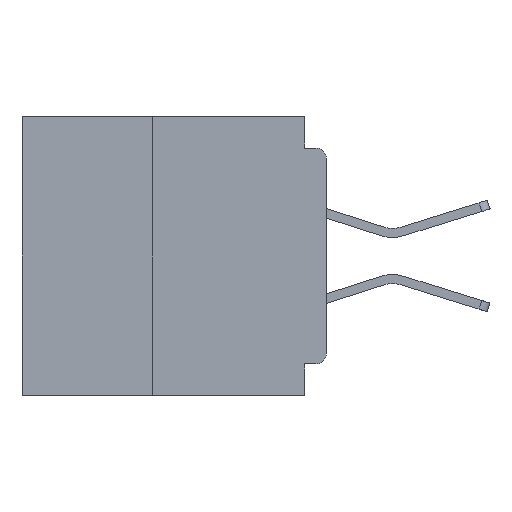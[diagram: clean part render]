
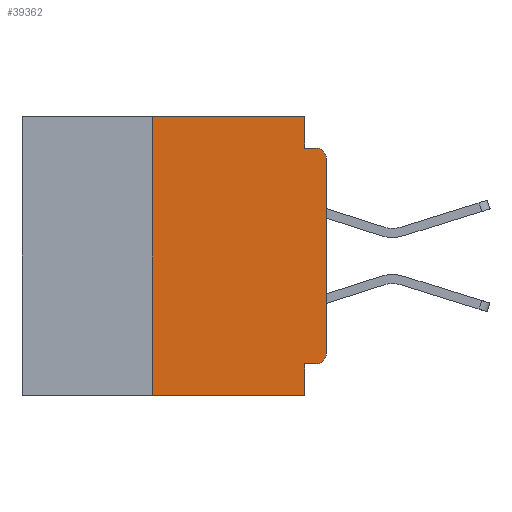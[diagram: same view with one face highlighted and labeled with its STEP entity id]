
A CAD part, left-side view. The second image highlights one B-rep face of the part: STEP entity #39362.
In plain terms, the highlighted planar face has unit normal (-1, 0, 0).
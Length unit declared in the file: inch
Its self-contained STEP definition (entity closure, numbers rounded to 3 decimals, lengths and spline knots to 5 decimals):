
#605 = DIRECTION ( 'NONE',  ( -1., 0., 0. ) ) ;
#1398 = CARTESIAN_POINT ( 'NONE',  ( 0., 0.25, 0. ) ) ;
#1966 = EDGE_CURVE ( 'NONE', #12375, #39930, #5953, .T. ) ;
#2686 = CARTESIAN_POINT ( 'NONE',  ( 0., 0., 0. ) ) ;
#2835 = ORIENTED_EDGE ( 'NONE', *, *, #18315, .T. ) ;
#3194 = DIRECTION ( 'NONE',  ( 0., 1., 0. ) ) ;
#5110 = CARTESIAN_POINT ( 'NONE',  ( 0., 0.25, -0.4 ) ) ;
#5703 = LINE ( 'NONE', #2686, #30418 ) ;
#5946 = AXIS2_PLACEMENT_3D ( 'NONE', #6601, #29172, #9844 ) ;
#5953 = LINE ( 'NONE', #39420, #28648 ) ;
#6601 = CARTESIAN_POINT ( 'NONE',  ( 0., 0.015, -0.34 ) ) ;
#7279 = ORIENTED_EDGE ( 'NONE', *, *, #30852, .F. ) ;
#7364 = PLANE ( 'NONE',  #23632 ) ;
#9844 = DIRECTION ( 'NONE',  ( 0., 0., -1. ) ) ;
#10402 = VECTOR ( 'NONE', #3194, 39.37008 ) ;
#10815 = EDGE_CURVE ( 'NONE', #17379, #29961, #40975, .T. ) ;
#10957 = ORIENTED_EDGE ( 'NONE', *, *, #1966, .T. ) ;
#11171 = ORIENTED_EDGE ( 'NONE', *, *, #10815, .T. ) ;
#11207 = EDGE_CURVE ( 'NONE', #12375, #24664, #19325, .T. ) ;
#12375 = VERTEX_POINT ( 'NONE', #5110 ) ;
#13879 = DIRECTION ( 'NONE',  ( 0., 0., -1. ) ) ;
#14001 = VECTOR ( 'NONE', #37225, 39.37008 ) ;
#14435 = ORIENTED_EDGE ( 'NONE', *, *, #35117, .F. ) ;
#15140 = CARTESIAN_POINT ( 'NONE',  ( 0., 0., -0.34 ) ) ;
#15181 = ORIENTED_EDGE ( 'NONE', *, *, #16352, .F. ) ;
#15329 = VERTEX_POINT ( 'NONE', #35336 ) ;
#15531 = CIRCLE ( 'NONE', #5946, 0.015 ) ;
#15926 = FACE_OUTER_BOUND ( 'NONE', #25054, .T. ) ;
#16352 = EDGE_CURVE ( 'NONE', #31308, #29961, #40665, .T. ) ;
#17379 = VERTEX_POINT ( 'NONE', #39952 ) ;
#18208 = VERTEX_POINT ( 'NONE', #15140 ) ;
#18305 = VECTOR ( 'NONE', #28153, 39.37008 ) ;
#18315 = EDGE_CURVE ( 'NONE', #18208, #17379, #5703, .T. ) ;
#18844 = VECTOR ( 'NONE', #39187, 39.37008 ) ;
#19325 = LINE ( 'NONE', #24911, #18305 ) ;
#19331 = CARTESIAN_POINT ( 'NONE',  ( 0., 0.031, -0.045 ) ) ;
#19873 = CARTESIAN_POINT ( 'NONE',  ( 0., 0.031, -0.4 ) ) ;
#19899 = CARTESIAN_POINT ( 'NONE',  ( 0., 0.015, -0.06 ) ) ;
#22555 = EDGE_CURVE ( 'NONE', #22811, #18208, #15531, .T. ) ;
#22563 = ORIENTED_EDGE ( 'NONE', *, *, #11207, .F. ) ;
#22811 = VERTEX_POINT ( 'NONE', #23915 ) ;
#23142 = DIRECTION ( 'NONE',  ( 0., 0., -1. ) ) ;
#23632 = AXIS2_PLACEMENT_3D ( 'NONE', #29913, #33124, #13879 ) ;
#23915 = CARTESIAN_POINT ( 'NONE',  ( 0., 0.015, -0.355 ) ) ;
#24546 = DIRECTION ( 'NONE',  ( 0., -1., 0. ) ) ;
#24607 = VECTOR ( 'NONE', #32997, 39.37008 ) ;
#24664 = VERTEX_POINT ( 'NONE', #1398 ) ;
#24735 = CARTESIAN_POINT ( 'NONE',  ( 0., 0.015, -0.045 ) ) ;
#24911 = CARTESIAN_POINT ( 'NONE',  ( 0., 0.25, -0.4 ) ) ;
#25054 = EDGE_LOOP ( 'NONE', ( #2835, #11171, #15181, #36501, #30398, #22563, #10957, #7279, #14435, #37507 ) ) ;
#25589 = LINE ( 'NONE', #29792, #24607 ) ;
#25751 = CARTESIAN_POINT ( 'NONE',  ( 0., 0.031, 0. ) ) ;
#27282 = VECTOR ( 'NONE', #24546, 39.37008 ) ;
#28153 = DIRECTION ( 'NONE',  ( 0., 0., 1. ) ) ;
#28418 = LINE ( 'NONE', #35930, #18844 ) ;
#28648 = VECTOR ( 'NONE', #38676, 39.37008 ) ;
#28766 = EDGE_CURVE ( 'NONE', #24664, #39794, #35855, .T. ) ;
#29172 = DIRECTION ( 'NONE',  ( -1., 0., 0. ) ) ;
#29792 = CARTESIAN_POINT ( 'NONE',  ( 0., 0.031, -0.4 ) ) ;
#29913 = CARTESIAN_POINT ( 'NONE',  ( 0., 0.437, 0. ) ) ;
#29961 = VERTEX_POINT ( 'NONE', #24735 ) ;
#30398 = ORIENTED_EDGE ( 'NONE', *, *, #28766, .F. ) ;
#30418 = VECTOR ( 'NONE', #34918, 39.37008 ) ;
#30852 = EDGE_CURVE ( 'NONE', #15329, #39930, #25589, .T. ) ;
#31308 = VERTEX_POINT ( 'NONE', #19331 ) ;
#32997 = DIRECTION ( 'NONE',  ( 0., 0., -1. ) ) ;
#33124 = DIRECTION ( 'NONE',  ( 1., 0., 0. ) ) ;
#33962 = CARTESIAN_POINT ( 'NONE',  ( 0., 0., -0.045 ) ) ;
#34918 = DIRECTION ( 'NONE',  ( 0., 0., 1. ) ) ;
#35049 = LINE ( 'NONE', #38547, #10402 ) ;
#35117 = EDGE_CURVE ( 'NONE', #22811, #15329, #35049, .T. ) ;
#35336 = CARTESIAN_POINT ( 'NONE',  ( 0., 0.031, -0.355 ) ) ;
#35855 = LINE ( 'NONE', #40579, #27282 ) ;
#35930 = CARTESIAN_POINT ( 'NONE',  ( 0., 0.031, 0. ) ) ;
#36501 = ORIENTED_EDGE ( 'NONE', *, *, #37078, .F. ) ;
#37078 = EDGE_CURVE ( 'NONE', #39794, #31308, #28418, .T. ) ;
#37225 = DIRECTION ( 'NONE',  ( 0., -1., 0. ) ) ;
#37233 = AXIS2_PLACEMENT_3D ( 'NONE', #19899, #605, #23142 ) ;
#37507 = ORIENTED_EDGE ( 'NONE', *, *, #22555, .T. ) ;
#38547 = CARTESIAN_POINT ( 'NONE',  ( 0., 0., -0.355 ) ) ;
#38676 = DIRECTION ( 'NONE',  ( 0., -1., 0. ) ) ;
#39187 = DIRECTION ( 'NONE',  ( 0., 0., -1. ) ) ;
#39362 = ADVANCED_FACE ( 'NONE', ( #15926 ), #7364, .F. ) ;
#39420 = CARTESIAN_POINT ( 'NONE',  ( 0., 0.437, -0.4 ) ) ;
#39794 = VERTEX_POINT ( 'NONE', #25751 ) ;
#39930 = VERTEX_POINT ( 'NONE', #19873 ) ;
#39952 = CARTESIAN_POINT ( 'NONE',  ( 0., 0., -0.06 ) ) ;
#40579 = CARTESIAN_POINT ( 'NONE',  ( 0., 0.437, 0. ) ) ;
#40665 = LINE ( 'NONE', #33962, #14001 ) ;
#40975 = CIRCLE ( 'NONE', #37233, 0.015 ) ;
